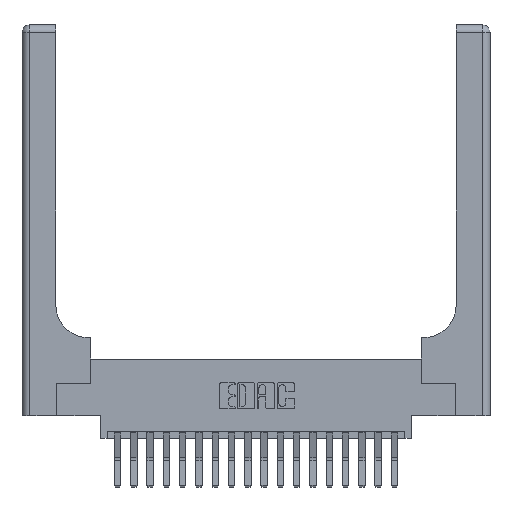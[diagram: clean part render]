
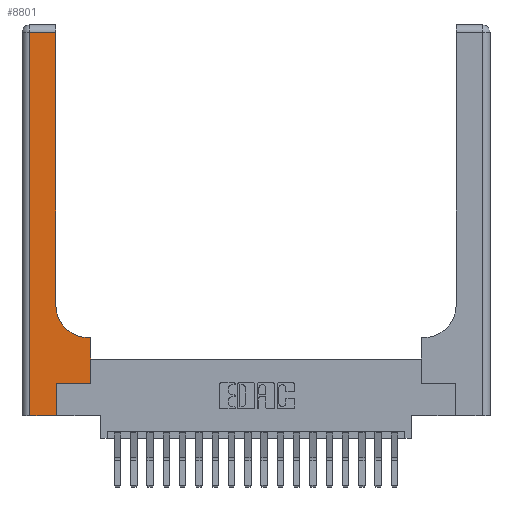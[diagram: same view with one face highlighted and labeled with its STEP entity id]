
A CAD part, top view. The second image highlights one B-rep face of the part: STEP entity #8801.
In plain terms, the highlighted planar face has unit normal (0, 0, 1).
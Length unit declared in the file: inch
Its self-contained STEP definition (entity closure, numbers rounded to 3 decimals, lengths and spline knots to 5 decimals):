
#288 = DIRECTION ( 'NONE',  ( 1., 0., 0. ) ) ;
#973 = ORIENTED_EDGE ( 'NONE', *, *, #2479, .T. ) ;
#1015 = VECTOR ( 'NONE', #12450, 39.37008 ) ;
#1080 = ORIENTED_EDGE ( 'NONE', *, *, #6022, .T. ) ;
#1267 = CARTESIAN_POINT ( 'NONE',  ( 0., 2.94, 0.37 ) ) ;
#1333 = DIRECTION ( 'NONE',  ( 0., 1., 0. ) ) ;
#1459 = CARTESIAN_POINT ( 'NONE',  ( 0.06, 3., 0.37 ) ) ;
#1542 = CARTESIAN_POINT ( 'NONE',  ( 0.528, 0.25, 0.37 ) ) ;
#1968 = ORIENTED_EDGE ( 'NONE', *, *, #8823, .T. ) ;
#2068 = ORIENTED_EDGE ( 'NONE', *, *, #2441, .T. ) ;
#2315 = DIRECTION ( 'NONE',  ( 0., 0., -1. ) ) ;
#2360 = EDGE_CURVE ( 'NONE', #9903, #10446, #20789, .T. ) ;
#2441 = EDGE_CURVE ( 'NONE', #13726, #11577, #2856, .T. ) ;
#2479 = EDGE_CURVE ( 'NONE', #10364, #8316, #12064, .T. ) ;
#2639 = DIRECTION ( 'NONE',  ( -1., 0., 0. ) ) ;
#2754 = DIRECTION ( 'NONE',  ( 1., 0., 0. ) ) ;
#2856 = LINE ( 'NONE', #1267, #11038 ) ;
#3067 = VECTOR ( 'NONE', #17749, 39.37008 ) ;
#3377 = CARTESIAN_POINT ( 'NONE',  ( 0.51, 0.6, 0.37 ) ) ;
#3515 = EDGE_CURVE ( 'NONE', #10446, #10810, #19303, .T. ) ;
#3609 = ORIENTED_EDGE ( 'NONE', *, *, #5126, .T. ) ;
#3734 = VECTOR ( 'NONE', #1333, 39.37008 ) ;
#4637 = CARTESIAN_POINT ( 'NONE',  ( 0.06, 0., 0.37 ) ) ;
#5020 = EDGE_CURVE ( 'NONE', #16451, #10501, #15985, .T. ) ;
#5119 = VECTOR ( 'NONE', #2639, 39.37008 ) ;
#5126 = EDGE_CURVE ( 'NONE', #10810, #16451, #9827, .T. ) ;
#5881 = DIRECTION ( 'NONE',  ( 0., 0., -1. ) ) ;
#6022 = EDGE_CURVE ( 'NONE', #11577, #9903, #20664, .T. ) ;
#6025 = CARTESIAN_POINT ( 'NONE',  ( 0.26, 2.94, 0.37 ) ) ;
#6080 = CARTESIAN_POINT ( 'NONE',  ( 0.26, 0.6, 0.37 ) ) ;
#6194 = DIRECTION ( 'NONE',  ( -1., 0., 0. ) ) ;
#6487 = ORIENTED_EDGE ( 'NONE', *, *, #3515, .T. ) ;
#6742 = CARTESIAN_POINT ( 'NONE',  ( 0.265, 0., 0.37 ) ) ;
#7764 = LINE ( 'NONE', #6080, #5119 ) ;
#8316 = VERTEX_POINT ( 'NONE', #13614 ) ;
#8333 = AXIS2_PLACEMENT_3D ( 'NONE', #10508, #2315, #18558 ) ;
#8801 = ADVANCED_FACE ( 'NONE', ( #17298 ), #18782, .F. ) ;
#8823 = EDGE_CURVE ( 'NONE', #10501, #10364, #7764, .T. ) ;
#9348 = CARTESIAN_POINT ( 'NONE',  ( 0., 3., 0.37 ) ) ;
#9687 = ORIENTED_EDGE ( 'NONE', *, *, #2360, .T. ) ;
#9756 = DIRECTION ( 'NONE',  ( -1., 0., 0. ) ) ;
#9827 = LINE ( 'NONE', #16313, #11825 ) ;
#9903 = VERTEX_POINT ( 'NONE', #4637 ) ;
#10364 = VERTEX_POINT ( 'NONE', #3377 ) ;
#10446 = VERTEX_POINT ( 'NONE', #6742 ) ;
#10501 = VERTEX_POINT ( 'NONE', #16986 ) ;
#10508 = CARTESIAN_POINT ( 'NONE',  ( 0.51, 0.85, 0.37 ) ) ;
#10810 = VERTEX_POINT ( 'NONE', #13321 ) ;
#11038 = VECTOR ( 'NONE', #9756, 39.37008 ) ;
#11129 = DIRECTION ( 'NONE',  ( 0., -1., 0. ) ) ;
#11577 = VERTEX_POINT ( 'NONE', #14521 ) ;
#11825 = VECTOR ( 'NONE', #288, 39.37008 ) ;
#12064 = CIRCLE ( 'NONE', #8333, 0.25 ) ;
#12066 = ORIENTED_EDGE ( 'NONE', *, *, #5020, .T. ) ;
#12450 = DIRECTION ( 'NONE',  ( 0., 1., 0. ) ) ;
#12499 = VECTOR ( 'NONE', #11129, 39.37008 ) ;
#13321 = CARTESIAN_POINT ( 'NONE',  ( 0.265, 0.25, 0.37 ) ) ;
#13614 = CARTESIAN_POINT ( 'NONE',  ( 0.26, 0.85, 0.37 ) ) ;
#13726 = VERTEX_POINT ( 'NONE', #6025 ) ;
#14521 = CARTESIAN_POINT ( 'NONE',  ( 0.06, 2.94, 0.37 ) ) ;
#14892 = AXIS2_PLACEMENT_3D ( 'NONE', #9348, #5881, #6194 ) ;
#15985 = LINE ( 'NONE', #1542, #3734 ) ;
#16313 = CARTESIAN_POINT ( 'NONE',  ( 0.265, 0.25, 0.37 ) ) ;
#16451 = VERTEX_POINT ( 'NONE', #16913 ) ;
#16846 = EDGE_LOOP ( 'NONE', ( #20780, #2068, #1080, #9687, #6487, #3609, #12066, #1968, #973 ) ) ;
#16913 = CARTESIAN_POINT ( 'NONE',  ( 0.528, 0.25, 0.37 ) ) ;
#16986 = CARTESIAN_POINT ( 'NONE',  ( 0.528, 0.6, 0.37 ) ) ;
#17298 = FACE_OUTER_BOUND ( 'NONE', #16846, .T. ) ;
#17602 = CARTESIAN_POINT ( 'NONE',  ( 0., 0., 0.37 ) ) ;
#17749 = DIRECTION ( 'NONE',  ( 0., 1., 0. ) ) ;
#18558 = DIRECTION ( 'NONE',  ( 1., 0., 0. ) ) ;
#18766 = EDGE_CURVE ( 'NONE', #8316, #13726, #19316, .T. ) ;
#18782 = PLANE ( 'NONE',  #14892 ) ;
#18825 = CARTESIAN_POINT ( 'NONE',  ( 0.265, 0., 0.37 ) ) ;
#19303 = LINE ( 'NONE', #18825, #1015 ) ;
#19316 = LINE ( 'NONE', #20709, #3067 ) ;
#19842 = VECTOR ( 'NONE', #2754, 39.37008 ) ;
#20664 = LINE ( 'NONE', #1459, #12499 ) ;
#20709 = CARTESIAN_POINT ( 'NONE',  ( 0.26, 3., 0.37 ) ) ;
#20780 = ORIENTED_EDGE ( 'NONE', *, *, #18766, .T. ) ;
#20789 = LINE ( 'NONE', #17602, #19842 ) ;
